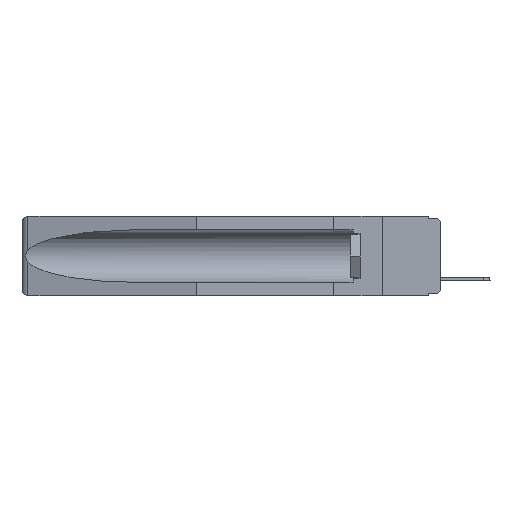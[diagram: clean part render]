
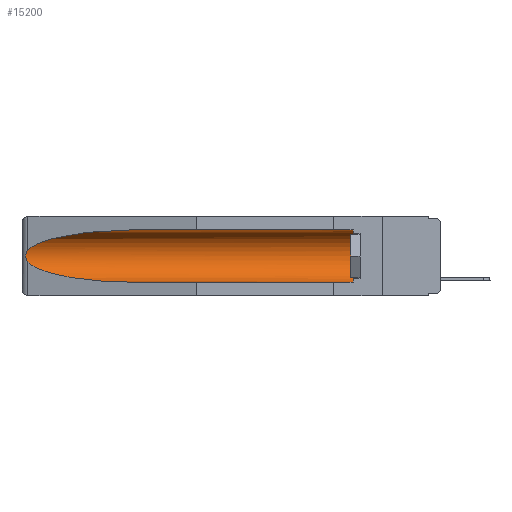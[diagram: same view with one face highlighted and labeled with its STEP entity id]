
A CAD part, left-side view. The second image highlights one B-rep face of the part: STEP entity #15200.
In plain terms, the highlighted cylindrical face has radius 2.857 mm (diameter 5.715 mm), a partial arc.
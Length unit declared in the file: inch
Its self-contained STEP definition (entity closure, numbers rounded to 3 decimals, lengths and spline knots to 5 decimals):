
#178 = CARTESIAN_POINT ( 'NONE',  ( 0.155, 1.07973, -0.284 ) ) ;
#350 = CARTESIAN_POINT ( 'NONE',  ( 0.2673, 1.5327, -0.16383 ) ) ;
#625 = VERTEX_POINT ( 'NONE', #16043 ) ;
#1456 = CARTESIAN_POINT ( 'NONE',  ( 0.155, 0.126, -0.284 ) ) ;
#1616 = CARTESIAN_POINT ( 'NONE',  ( 0.26537, 1.52718, -0.19328 ) ) ;
#2374 = VERTEX_POINT ( 'NONE', #178 ) ;
#3963 = VERTEX_POINT ( 'NONE', #1456 ) ;
#4363 = CARTESIAN_POINT ( 'NONE',  ( 0.2673, 1.53269, -0.17917 ) ) ;
#4638 = CARTESIAN_POINT ( 'NONE',  ( 0.2675, 1.53308, -0.17534 ) ) ;
#5256 = EDGE_CURVE ( 'NONE', #625, #6998, #21075, .T. ) ;
#5507 = CARTESIAN_POINT ( 'NONE',  ( 0.155, -0.30754, -0.059 ) ) ;
#5620 = CARTESIAN_POINT ( 'NONE',  ( 0.26537, 1.52718, -0.14972 ) ) ;
#5664 = EDGE_LOOP ( 'NONE', ( #9987, #17832, #13553, #15454, #14226, #12695 ) ) ;
#6181 = CARTESIAN_POINT ( 'NONE',  ( 0.25451, 1.48313, -0.24835 ) ) ;
#6836 = CARTESIAN_POINT ( 'NONE',  ( 0.155, 0.126, -0.1715 ) ) ;
#6998 = VERTEX_POINT ( 'NONE', #25210 ) ;
#7430 = EDGE_CURVE ( 'NONE', #3963, #2374, #12892, .T. ) ;
#8360 = CARTESIAN_POINT ( 'NONE',  ( 0.155, 1.07973, -0.059 ) ) ;
#9525 = CIRCLE ( 'NONE', #21373, 0.1125 ) ;
#9922 = CARTESIAN_POINT ( 'NONE',  ( 0.26537, 1.52718, -0.19328 ) ) ;
#9987 = ORIENTED_EDGE ( 'NONE', *, *, #18658, .T. ) ;
#10201 = CYLINDRICAL_SURFACE ( 'NONE', #25404, 0.1125 ) ;
#10614 = DIRECTION ( 'NONE',  ( 0., 1., 0. ) ) ;
#11697 = EDGE_CURVE ( 'NONE', #24089, #17372, #14072, .T. ) ;
#12478 = FACE_OUTER_BOUND ( 'NONE', #5664, .T. ) ;
#12695 = ORIENTED_EDGE ( 'NONE', *, *, #5256, .T. ) ;
#12892 = LINE ( 'NONE', #23477, #14340 ) ;
#12916 = CARTESIAN_POINT ( 'NONE',  ( 0.25451, 1.48313, -0.09465 ) ) ;
#13226 = CARTESIAN_POINT ( 'NONE',  ( 0.26537, 1.52718, -0.14972 ) ) ;
#13505 = CARTESIAN_POINT ( 'NONE',  ( 0.26655, 1.53094, -0.18657 ) ) ;
#13553 = ORIENTED_EDGE ( 'NONE', *, *, #21677, .T. ) ;
#14072 = B_SPLINE_CURVE_WITH_KNOTS ( 'NONE', 3,
 ( #13226, #17506, #15522, #350, #22081, #4638, #4363, #13505, #15110, #21651 ),
 .UNSPECIFIED., .F., .F.,
 ( 4, 2, 2, 2, 4 ),
 ( 0., 0.00029, 0.00058, 0.00087, 0.00117 ),
 .UNSPECIFIED. ) ;
#14226 = ORIENTED_EDGE ( 'NONE', *, *, #17792, .T. ) ;
#14340 = VECTOR ( 'NONE', #10614, 39.37008 ) ;
#14925 = DIRECTION ( 'NONE',  ( 0., 1., 0. ) ) ;
#15110 = CARTESIAN_POINT ( 'NONE',  ( 0.26597, 1.5296, -0.19026 ) ) ;
#15200 = ADVANCED_FACE ( 'NONE', ( #12478 ), #10201, .F. ) ;
#15454 = ORIENTED_EDGE ( 'NONE', *, *, #7430, .F. ) ;
#15522 = CARTESIAN_POINT ( 'NONE',  ( 0.26654, 1.53092, -0.15636 ) ) ;
#15555 = DIRECTION ( 'NONE',  ( 0., 0., 1. ) ) ;
#16043 = CARTESIAN_POINT ( 'NONE',  ( 0.155, 0.126, -0.059 ) ) ;
#16378 =( BOUNDED_CURVE ( )  B_SPLINE_CURVE ( 3, ( #9922, #6181, #18752, #21464 ),
 .UNSPECIFIED., .F., .F. ) 
 B_SPLINE_CURVE_WITH_KNOTS ( ( 4, 4 ),
 ( 0.1948, 1.5708 ),
 .UNSPECIFIED. ) 
 CURVE ( )  GEOMETRIC_REPRESENTATION_ITEM ( )  RATIONAL_B_SPLINE_CURVE ( ( 1., 0.848, 0.848, 1. ) ) 
 REPRESENTATION_ITEM ( '' )  );
#17372 = VERTEX_POINT ( 'NONE', #1616 ) ;
#17506 = CARTESIAN_POINT ( 'NONE',  ( 0.26597, 1.52961, -0.15275 ) ) ;
#17792 = EDGE_CURVE ( 'NONE', #3963, #625, #9525, .T. ) ;
#17832 = ORIENTED_EDGE ( 'NONE', *, *, #11697, .T. ) ;
#18658 = EDGE_CURVE ( 'NONE', #6998, #24089, #28045, .T. ) ;
#18752 = CARTESIAN_POINT ( 'NONE',  ( 0.21114, 1.30732, -0.284 ) ) ;
#18889 = DIRECTION ( 'NONE',  ( 0., 0., 1. ) ) ;
#21075 = LINE ( 'NONE', #5507, #22721 ) ;
#21188 = CARTESIAN_POINT ( 'NONE',  ( 0.155, -0.30754, -0.1715 ) ) ;
#21373 = AXIS2_PLACEMENT_3D ( 'NONE', #6836, #24125, #15555 ) ;
#21464 = CARTESIAN_POINT ( 'NONE',  ( 0.155, 1.07973, -0.284 ) ) ;
#21651 = CARTESIAN_POINT ( 'NONE',  ( 0.26537, 1.52718, -0.19328 ) ) ;
#21677 = EDGE_CURVE ( 'NONE', #17372, #2374, #16378, .T. ) ;
#22081 = CARTESIAN_POINT ( 'NONE',  ( 0.2675, 1.53308, -0.16763 ) ) ;
#22721 = VECTOR ( 'NONE', #23239, 39.37008 ) ;
#23239 = DIRECTION ( 'NONE',  ( 0., 1., 0. ) ) ;
#23477 = CARTESIAN_POINT ( 'NONE',  ( 0.155, -0.30754, -0.284 ) ) ;
#23783 = CARTESIAN_POINT ( 'NONE',  ( 0.21114, 1.30732, -0.059 ) ) ;
#23917 = CARTESIAN_POINT ( 'NONE',  ( 0.26537, 1.52718, -0.14972 ) ) ;
#24089 = VERTEX_POINT ( 'NONE', #5620 ) ;
#24125 = DIRECTION ( 'NONE',  ( 0., -1., 0. ) ) ;
#25210 = CARTESIAN_POINT ( 'NONE',  ( 0.155, 1.07973, -0.059 ) ) ;
#25404 = AXIS2_PLACEMENT_3D ( 'NONE', #21188, #14925, #18889 ) ;
#28045 =( BOUNDED_CURVE ( )  B_SPLINE_CURVE ( 3, ( #8360, #23783, #12916, #23917 ),
 .UNSPECIFIED., .F., .F. ) 
 B_SPLINE_CURVE_WITH_KNOTS ( ( 4, 4 ),
 ( 4.71239, 6.08839 ),
 .UNSPECIFIED. ) 
 CURVE ( )  GEOMETRIC_REPRESENTATION_ITEM ( )  RATIONAL_B_SPLINE_CURVE ( ( 1., 0.848, 0.848, 1. ) ) 
 REPRESENTATION_ITEM ( '' )  );
